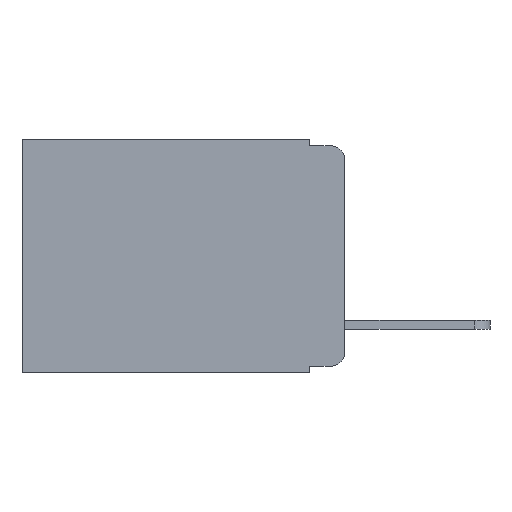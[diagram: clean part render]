
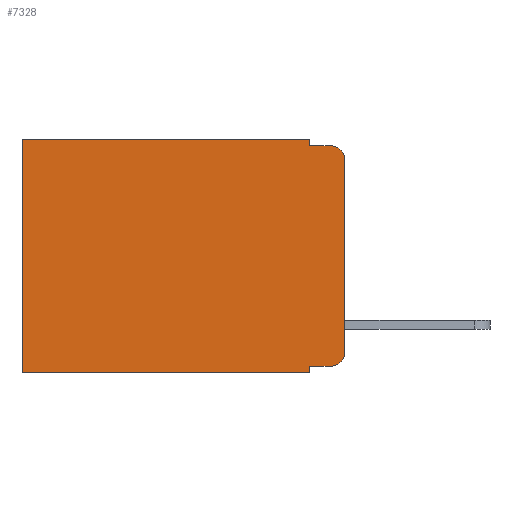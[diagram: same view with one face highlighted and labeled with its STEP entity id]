
A CAD part, left-side view. The second image highlights one B-rep face of the part: STEP entity #7328.
In plain terms, the highlighted planar face has unit normal (-1, 0, 0).
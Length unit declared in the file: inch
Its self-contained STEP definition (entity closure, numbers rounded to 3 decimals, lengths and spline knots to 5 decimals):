
#17 = DIRECTION ( 'NONE',  ( 0., 0., -1. ) ) ;
#37 = DIRECTION ( 'NONE',  ( -1., 0., 0. ) ) ;
#390 = ORIENTED_EDGE ( 'NONE', *, *, #14058, .F. ) ;
#633 = CARTESIAN_POINT ( 'NONE',  ( 0.298, 0.051, 0. ) ) ;
#909 = EDGE_CURVE ( 'NONE', #8341, #19046, #15987, .T. ) ;
#991 = DIRECTION ( 'NONE',  ( -1., 0., 0. ) ) ;
#1121 = CARTESIAN_POINT ( 'NONE',  ( 0.298, 0.051, 0. ) ) ;
#1198 = CARTESIAN_POINT ( 'NONE',  ( 0.298, 0., 0. ) ) ;
#1321 = PLANE ( 'NONE',  #15466 ) ;
#1540 = CARTESIAN_POINT ( 'NONE',  ( 0.298, 0.051, 0. ) ) ;
#1656 = LINE ( 'NONE', #17539, #8521 ) ;
#1672 = DIRECTION ( 'NONE',  ( 0., 0., -1. ) ) ;
#1859 = CARTESIAN_POINT ( 'NONE',  ( 0.298, 0.02, -0.333 ) ) ;
#2645 = EDGE_CURVE ( 'NONE', #6091, #3103, #3918, .T. ) ;
#2732 = LINE ( 'NONE', #9261, #5043 ) ;
#2790 = DIRECTION ( 'NONE',  ( 0., 0., -1. ) ) ;
#2822 = ORIENTED_EDGE ( 'NONE', *, *, #8375, .T. ) ;
#3054 = VERTEX_POINT ( 'NONE', #17164 ) ;
#3103 = VERTEX_POINT ( 'NONE', #17528 ) ;
#3175 = ORIENTED_EDGE ( 'NONE', *, *, #9797, .T. ) ;
#3240 = LINE ( 'NONE', #633, #5774 ) ;
#3314 = EDGE_CURVE ( 'NONE', #20117, #10756, #1656, .T. ) ;
#3413 = VECTOR ( 'NONE', #17, 39.37008 ) ;
#3918 = LINE ( 'NONE', #12961, #3413 ) ;
#4502 = EDGE_CURVE ( 'NONE', #10720, #16906, #12790, .T. ) ;
#4859 = DIRECTION ( 'NONE',  ( 0., 0., -1. ) ) ;
#5043 = VECTOR ( 'NONE', #2790, 39.37008 ) ;
#5088 = DIRECTION ( 'NONE',  ( 0., -1., 0. ) ) ;
#5774 = VECTOR ( 'NONE', #8534, 39.37008 ) ;
#6062 = DIRECTION ( 'NONE',  ( 0., -1., 0. ) ) ;
#6091 = VERTEX_POINT ( 'NONE', #13628 ) ;
#6319 = VECTOR ( 'NONE', #4859, 39.37008 ) ;
#6372 = EDGE_CURVE ( 'NONE', #19651, #10756, #2732, .T. ) ;
#6970 = LINE ( 'NONE', #1198, #20671 ) ;
#7328 = ADVANCED_FACE ( 'NONE', ( #9034 ), #1321, .F. ) ;
#7782 = DIRECTION ( 'NONE',  ( 0., 1., 0. ) ) ;
#8341 = VERTEX_POINT ( 'NONE', #1121 ) ;
#8375 = EDGE_CURVE ( 'NONE', #8341, #19651, #6970, .T. ) ;
#8376 = ORIENTED_EDGE ( 'NONE', *, *, #4502, .T. ) ;
#8521 = VECTOR ( 'NONE', #7782, 39.37008 ) ;
#8534 = DIRECTION ( 'NONE',  ( 0., 0., -1. ) ) ;
#9034 = FACE_OUTER_BOUND ( 'NONE', #13087, .T. ) ;
#9261 = CARTESIAN_POINT ( 'NONE',  ( 0.298, 0.473, 0. ) ) ;
#9797 = EDGE_CURVE ( 'NONE', #6091, #3054, #19260, .T. ) ;
#10273 = EDGE_CURVE ( 'NONE', #19046, #3054, #15703, .T. ) ;
#10720 = VERTEX_POINT ( 'NONE', #15503 ) ;
#10756 = VERTEX_POINT ( 'NONE', #18625 ) ;
#12277 = ORIENTED_EDGE ( 'NONE', *, *, #3314, .F. ) ;
#12367 = DIRECTION ( 'NONE',  ( 0., 0., -1. ) ) ;
#12426 = DIRECTION ( 'NONE',  ( 0., 0., -1. ) ) ;
#12790 = LINE ( 'NONE', #17880, #17624 ) ;
#12961 = CARTESIAN_POINT ( 'NONE',  ( 0.298, 0., 0. ) ) ;
#13087 = EDGE_LOOP ( 'NONE', ( #17832, #3175, #14401, #13623, #2822, #13234, #12277, #390, #8376, #16842 ) ) ;
#13234 = ORIENTED_EDGE ( 'NONE', *, *, #6372, .T. ) ;
#13623 = ORIENTED_EDGE ( 'NONE', *, *, #909, .F. ) ;
#13628 = CARTESIAN_POINT ( 'NONE',  ( 0.298, 0., -0.03 ) ) ;
#13963 = CARTESIAN_POINT ( 'NONE',  ( 0.298, 0.051, -0.01 ) ) ;
#13996 = AXIS2_PLACEMENT_3D ( 'NONE', #17882, #37, #1672 ) ;
#14058 = EDGE_CURVE ( 'NONE', #10720, #20117, #3240, .T. ) ;
#14181 = DIRECTION ( 'NONE',  ( 1., 0., 0. ) ) ;
#14306 = CARTESIAN_POINT ( 'NONE',  ( 0.298, 0.051, -0.01 ) ) ;
#14401 = ORIENTED_EDGE ( 'NONE', *, *, #10273, .F. ) ;
#14439 = CARTESIAN_POINT ( 'NONE',  ( 0.298, 0.473, 0. ) ) ;
#15466 = AXIS2_PLACEMENT_3D ( 'NONE', #17447, #14181, #12426 ) ;
#15503 = CARTESIAN_POINT ( 'NONE',  ( 0.298, 0.051, -0.333 ) ) ;
#15703 = LINE ( 'NONE', #13963, #17234 ) ;
#15851 = EDGE_CURVE ( 'NONE', #16906, #3103, #18828, .T. ) ;
#15987 = LINE ( 'NONE', #1540, #6319 ) ;
#16113 = AXIS2_PLACEMENT_3D ( 'NONE', #20426, #991, #12367 ) ;
#16842 = ORIENTED_EDGE ( 'NONE', *, *, #15851, .T. ) ;
#16906 = VERTEX_POINT ( 'NONE', #1859 ) ;
#17164 = CARTESIAN_POINT ( 'NONE',  ( 0.298, 0.02, -0.01 ) ) ;
#17234 = VECTOR ( 'NONE', #6062, 39.37008 ) ;
#17447 = CARTESIAN_POINT ( 'NONE',  ( 0.298, 0., 0. ) ) ;
#17528 = CARTESIAN_POINT ( 'NONE',  ( 0.298, 0., -0.313 ) ) ;
#17539 = CARTESIAN_POINT ( 'NONE',  ( 0.298, 0., -0.343 ) ) ;
#17624 = VECTOR ( 'NONE', #5088, 39.37008 ) ;
#17832 = ORIENTED_EDGE ( 'NONE', *, *, #2645, .F. ) ;
#17880 = CARTESIAN_POINT ( 'NONE',  ( 0.298, 0.051, -0.333 ) ) ;
#17882 = CARTESIAN_POINT ( 'NONE',  ( 0.298, 0.02, -0.03 ) ) ;
#18625 = CARTESIAN_POINT ( 'NONE',  ( 0.298, 0.473, -0.343 ) ) ;
#18828 = CIRCLE ( 'NONE', #16113, 0.02 ) ;
#18947 = CARTESIAN_POINT ( 'NONE',  ( 0.298, 0.051, -0.343 ) ) ;
#19046 = VERTEX_POINT ( 'NONE', #14306 ) ;
#19260 = CIRCLE ( 'NONE', #13996, 0.02 ) ;
#19651 = VERTEX_POINT ( 'NONE', #14439 ) ;
#20117 = VERTEX_POINT ( 'NONE', #18947 ) ;
#20426 = CARTESIAN_POINT ( 'NONE',  ( 0.298, 0.02, -0.313 ) ) ;
#20671 = VECTOR ( 'NONE', #20781, 39.37008 ) ;
#20781 = DIRECTION ( 'NONE',  ( 0., 1., 0. ) ) ;
